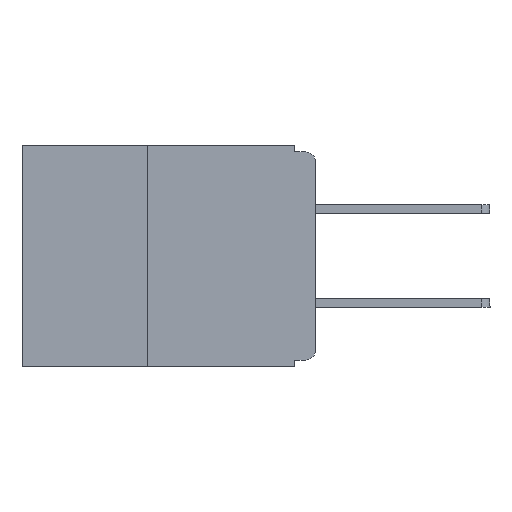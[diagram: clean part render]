
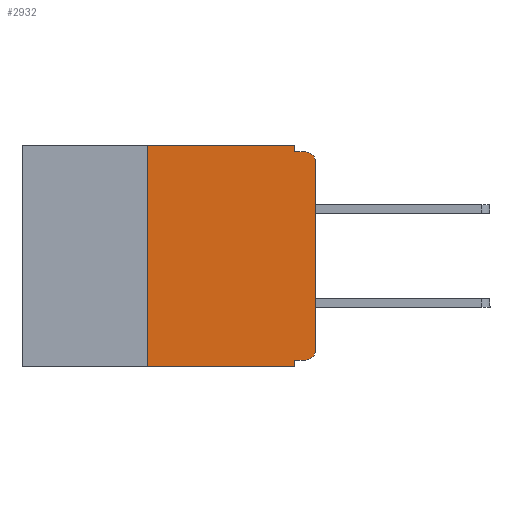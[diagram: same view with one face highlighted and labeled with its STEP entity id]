
A CAD part, left-side view. The second image highlights one B-rep face of the part: STEP entity #2932.
In plain terms, the highlighted planar face has unit normal (-1, 0, 0).
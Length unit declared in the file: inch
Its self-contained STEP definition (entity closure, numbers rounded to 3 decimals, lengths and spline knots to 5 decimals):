
#1000 = VERTEX_POINT ( 'NONE', #6044 ) ;
#1201 = FACE_OUTER_BOUND ( 'NONE', #11612, .T. ) ;
#1456 = VERTEX_POINT ( 'NONE', #12633 ) ;
#1930 = VERTEX_POINT ( 'NONE', #11860 ) ;
#2327 = VECTOR ( 'NONE', #2839, 39.37008 ) ;
#2353 = LINE ( 'NONE', #3722, #2327 ) ;
#2514 = EDGE_CURVE ( 'NONE', #3512, #10798, #2353, .T. ) ;
#2617 = DIRECTION ( 'NONE',  ( 0., 0., -1. ) ) ;
#2623 = DIRECTION ( 'NONE',  ( -1., 0., 0. ) ) ;
#2739 = VERTEX_POINT ( 'NONE', #5259 ) ;
#2839 = DIRECTION ( 'NONE',  ( 0., 0., -1. ) ) ;
#2866 = CARTESIAN_POINT ( 'NONE',  ( 0., 0.015, -0.305 ) ) ;
#2932 = ADVANCED_FACE ( 'NONE', ( #1201 ), #9661, .F. ) ;
#3403 = EDGE_CURVE ( 'NONE', #12846, #3512, #13173, .T. ) ;
#3472 = CIRCLE ( 'NONE', #6523, 0.015 ) ;
#3512 = VERTEX_POINT ( 'NONE', #4742 ) ;
#3578 = AXIS2_PLACEMENT_3D ( 'NONE', #5141, #4782, #4681 ) ;
#3659 = CIRCLE ( 'NONE', #3578, 0.015 ) ;
#3722 = CARTESIAN_POINT ( 'NONE',  ( 0., 0.031, 0. ) ) ;
#3838 = CARTESIAN_POINT ( 'NONE',  ( 0., 0.015, -0.32 ) ) ;
#4249 = VECTOR ( 'NONE', #12583, 39.37008 ) ;
#4476 = LINE ( 'NONE', #12570, #4249 ) ;
#4681 = DIRECTION ( 'NONE',  ( 0., 0., -1. ) ) ;
#4742 = CARTESIAN_POINT ( 'NONE',  ( 0., 0.031, 0. ) ) ;
#4782 = DIRECTION ( 'NONE',  ( -1., 0., 0. ) ) ;
#5141 = CARTESIAN_POINT ( 'NONE',  ( 0., 0.015, -0.025 ) ) ;
#5259 = CARTESIAN_POINT ( 'NONE',  ( 0., 0.015, -0.01 ) ) ;
#5796 = LINE ( 'NONE', #6986, #5885 ) ;
#5885 = VECTOR ( 'NONE', #6632, 39.37008 ) ;
#5946 = DIRECTION ( 'NONE',  ( 0., 0., 1. ) ) ;
#6044 = CARTESIAN_POINT ( 'NONE',  ( 0., 0.25, -0.33 ) ) ;
#6093 = CARTESIAN_POINT ( 'NONE',  ( 0., 0., 0. ) ) ;
#6179 = ORIENTED_EDGE ( 'NONE', *, *, #2514, .F. ) ;
#6202 = VECTOR ( 'NONE', #11245, 39.37008 ) ;
#6394 = AXIS2_PLACEMENT_3D ( 'NONE', #9061, #8454, #8403 ) ;
#6523 = AXIS2_PLACEMENT_3D ( 'NONE', #2866, #2623, #2617 ) ;
#6524 = CARTESIAN_POINT ( 'NONE',  ( 0., 0.437, -0.33 ) ) ;
#6611 = DIRECTION ( 'NONE',  ( 0., -1., 0. ) ) ;
#6620 = CARTESIAN_POINT ( 'NONE',  ( 0., 0.031, -0.01 ) ) ;
#6632 = DIRECTION ( 'NONE',  ( 0., -1., 0. ) ) ;
#6721 = ORIENTED_EDGE ( 'NONE', *, *, #3403, .F. ) ;
#6877 = LINE ( 'NONE', #11427, #6202 ) ;
#6956 = CARTESIAN_POINT ( 'NONE',  ( 0., 0.25, 0. ) ) ;
#6986 = CARTESIAN_POINT ( 'NONE',  ( 0., 0., -0.01 ) ) ;
#7127 = EDGE_CURVE ( 'NONE', #8095, #10411, #4476, .T. ) ;
#7361 = EDGE_CURVE ( 'NONE', #8864, #2739, #3659, .T. ) ;
#7408 = EDGE_CURVE ( 'NONE', #8095, #1930, #3472, .T. ) ;
#8095 = VERTEX_POINT ( 'NONE', #3838 ) ;
#8403 = DIRECTION ( 'NONE',  ( 0., 0., -1. ) ) ;
#8454 = DIRECTION ( 'NONE',  ( 1., 0., 0. ) ) ;
#8864 = VERTEX_POINT ( 'NONE', #12767 ) ;
#8968 = CARTESIAN_POINT ( 'NONE',  ( 0., 0.437, 0. ) ) ;
#9061 = CARTESIAN_POINT ( 'NONE',  ( 0., 0.437, 0. ) ) ;
#9062 = ORIENTED_EDGE ( 'NONE', *, *, #7361, .T. ) ;
#9338 = ORIENTED_EDGE ( 'NONE', *, *, #11403, .T. ) ;
#9486 = ORIENTED_EDGE ( 'NONE', *, *, #9663, .F. ) ;
#9547 = ORIENTED_EDGE ( 'NONE', *, *, #11538, .F. ) ;
#9555 = ORIENTED_EDGE ( 'NONE', *, *, #11376, .T. ) ;
#9617 = ORIENTED_EDGE ( 'NONE', *, *, #7127, .F. ) ;
#9631 = ORIENTED_EDGE ( 'NONE', *, *, #7408, .T. ) ;
#9661 = PLANE ( 'NONE',  #6394 ) ;
#9663 = EDGE_CURVE ( 'NONE', #1000, #12846, #6877, .T. ) ;
#9711 = VECTOR ( 'NONE', #12373, 39.37008 ) ;
#9743 = LINE ( 'NONE', #12586, #9711 ) ;
#10171 = VECTOR ( 'NONE', #6611, 39.37008 ) ;
#10210 = LINE ( 'NONE', #6524, #10171 ) ;
#10217 = ORIENTED_EDGE ( 'NONE', *, *, #12855, .F. ) ;
#10258 = LINE ( 'NONE', #6093, #10303 ) ;
#10303 = VECTOR ( 'NONE', #5946, 39.37008 ) ;
#10322 = DIRECTION ( 'NONE',  ( 0., -1., 0. ) ) ;
#10411 = VERTEX_POINT ( 'NONE', #11625 ) ;
#10798 = VERTEX_POINT ( 'NONE', #6620 ) ;
#11245 = DIRECTION ( 'NONE',  ( 0., 0., 1. ) ) ;
#11376 = EDGE_CURVE ( 'NONE', #1930, #8864, #10258, .T. ) ;
#11403 = EDGE_CURVE ( 'NONE', #1000, #1456, #10210, .T. ) ;
#11427 = CARTESIAN_POINT ( 'NONE',  ( 0., 0.25, -0.33 ) ) ;
#11538 = EDGE_CURVE ( 'NONE', #10411, #1456, #9743, .T. ) ;
#11612 = EDGE_LOOP ( 'NONE', ( #9555, #9062, #10217, #6179, #6721, #9486, #9338, #9547, #9617, #9631 ) ) ;
#11625 = CARTESIAN_POINT ( 'NONE',  ( 0., 0.031, -0.32 ) ) ;
#11860 = CARTESIAN_POINT ( 'NONE',  ( 0., 0., -0.305 ) ) ;
#12373 = DIRECTION ( 'NONE',  ( 0., 0., -1. ) ) ;
#12570 = CARTESIAN_POINT ( 'NONE',  ( 0., 0., -0.32 ) ) ;
#12583 = DIRECTION ( 'NONE',  ( 0., 1., 0. ) ) ;
#12586 = CARTESIAN_POINT ( 'NONE',  ( 0., 0.031, -0.33 ) ) ;
#12633 = CARTESIAN_POINT ( 'NONE',  ( 0., 0.031, -0.33 ) ) ;
#12767 = CARTESIAN_POINT ( 'NONE',  ( 0., 0., -0.025 ) ) ;
#12846 = VERTEX_POINT ( 'NONE', #6956 ) ;
#12855 = EDGE_CURVE ( 'NONE', #10798, #2739, #5796, .T. ) ;
#13022 = VECTOR ( 'NONE', #10322, 39.37008 ) ;
#13173 = LINE ( 'NONE', #8968, #13022 ) ;
